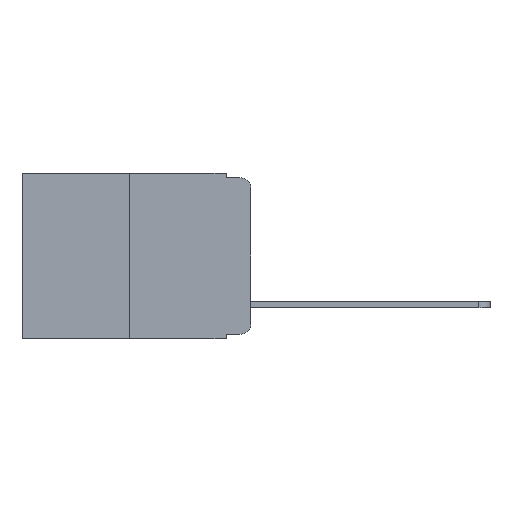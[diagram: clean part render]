
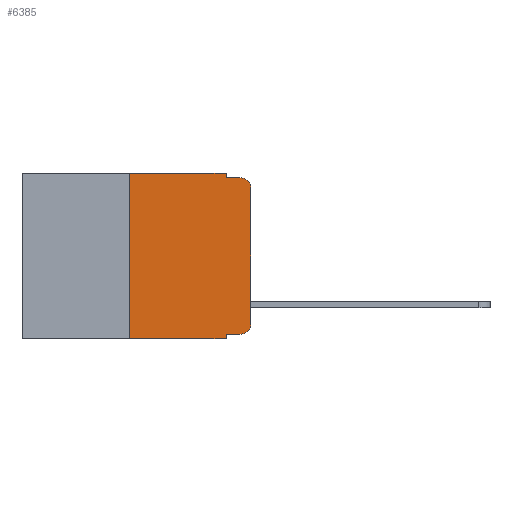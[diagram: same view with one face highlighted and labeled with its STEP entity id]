
A CAD part, left-side view. The second image highlights one B-rep face of the part: STEP entity #6385.
In plain terms, the highlighted planar face has unit normal (-1, 0, 0).
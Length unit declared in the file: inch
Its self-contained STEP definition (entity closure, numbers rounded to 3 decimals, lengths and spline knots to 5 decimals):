
#114 = VECTOR ( 'NONE', #10742, 39.37008 ) ;
#487 = ORIENTED_EDGE ( 'NONE', *, *, #7247, .T. ) ;
#564 = ORIENTED_EDGE ( 'NONE', *, *, #7189, .T. ) ;
#660 = ORIENTED_EDGE ( 'NONE', *, *, #6929, .F. ) ;
#783 = VERTEX_POINT ( 'NONE', #8067 ) ;
#1077 = ORIENTED_EDGE ( 'NONE', *, *, #7345, .T. ) ;
#1252 = ORIENTED_EDGE ( 'NONE', *, *, #6862, .F. ) ;
#1576 = VERTEX_POINT ( 'NONE', #7531 ) ;
#1654 = ORIENTED_EDGE ( 'NONE', *, *, #7230, .F. ) ;
#2025 = VERTEX_POINT ( 'NONE', #2436 ) ;
#2248 = DIRECTION ( 'NONE',  ( -1., 0., 0. ) ) ;
#2436 = CARTESIAN_POINT ( 'NONE',  ( 0., 0.02, -0.333 ) ) ;
#2529 = LINE ( 'NONE', #7719, #4609 ) ;
#2545 = ORIENTED_EDGE ( 'NONE', *, *, #6733, .F. ) ;
#2720 = CARTESIAN_POINT ( 'NONE',  ( 0., 0.051, 0. ) ) ;
#3143 = PLANE ( 'NONE',  #5312 ) ;
#3293 = CARTESIAN_POINT ( 'NONE',  ( 0., 0.051, -0.343 ) ) ;
#3547 = VECTOR ( 'NONE', #6724, 39.37008 ) ;
#3591 = ORIENTED_EDGE ( 'NONE', *, *, #5515, .T. ) ;
#3782 = AXIS2_PLACEMENT_3D ( 'NONE', #8034, #2248, #8924 ) ;
#3827 = DIRECTION ( 'NONE',  ( 0., 0., -1. ) ) ;
#4185 = VECTOR ( 'NONE', #3827, 39.37008 ) ;
#4446 = EDGE_LOOP ( 'NONE', ( #3591, #7866, #7164, #2545, #1654, #1252, #1077, #660, #564, #487 ) ) ;
#4468 = LINE ( 'NONE', #2720, #4185 ) ;
#4572 = VERTEX_POINT ( 'NONE', #9995 ) ;
#4609 = VECTOR ( 'NONE', #10327, 39.37008 ) ;
#4756 = LINE ( 'NONE', #7094, #9540 ) ;
#5075 = VECTOR ( 'NONE', #9643, 39.37008 ) ;
#5179 = DIRECTION ( 'NONE',  ( 0., 0., -1. ) ) ;
#5312 = AXIS2_PLACEMENT_3D ( 'NONE', #11291, #7882, #5179 ) ;
#5388 = LINE ( 'NONE', #6174, #5075 ) ;
#5488 = CARTESIAN_POINT ( 'NONE',  ( 0., 0.051, -0.01 ) ) ;
#5515 = EDGE_CURVE ( 'NONE', #6051, #1576, #6715, .T. ) ;
#5832 = LINE ( 'NONE', #9034, #114 ) ;
#5993 = DIRECTION ( 'NONE',  ( -1., 0., 0. ) ) ;
#6028 = VERTEX_POINT ( 'NONE', #11515 ) ;
#6043 = CARTESIAN_POINT ( 'NONE',  ( 0., 0.051, 0. ) ) ;
#6051 = VERTEX_POINT ( 'NONE', #8989 ) ;
#6174 = CARTESIAN_POINT ( 'NONE',  ( 0., 0.051, -0.333 ) ) ;
#6195 = EDGE_CURVE ( 'NONE', #1576, #6028, #8511, .T. ) ;
#6385 = ADVANCED_FACE ( 'NONE', ( #7403 ), #3143, .F. ) ;
#6624 = EDGE_CURVE ( 'NONE', #783, #6028, #12288, .T. ) ;
#6715 = LINE ( 'NONE', #11034, #10800 ) ;
#6724 = DIRECTION ( 'NONE',  ( 0., 0., 1. ) ) ;
#6733 = EDGE_CURVE ( 'NONE', #8177, #783, #4468, .T. ) ;
#6862 = EDGE_CURVE ( 'NONE', #7215, #4572, #10773, .T. ) ;
#6929 = EDGE_CURVE ( 'NONE', #12127, #11826, #2529, .T. ) ;
#7094 = CARTESIAN_POINT ( 'NONE',  ( 0., 0.473, 0. ) ) ;
#7164 = ORIENTED_EDGE ( 'NONE', *, *, #6624, .F. ) ;
#7189 = EDGE_CURVE ( 'NONE', #12127, #2025, #5388, .T. ) ;
#7215 = VERTEX_POINT ( 'NONE', #10550 ) ;
#7230 = EDGE_CURVE ( 'NONE', #4572, #8177, #4756, .T. ) ;
#7247 = EDGE_CURVE ( 'NONE', #2025, #6051, #9036, .T. ) ;
#7345 = EDGE_CURVE ( 'NONE', #7215, #11826, #5832, .T. ) ;
#7403 = FACE_OUTER_BOUND ( 'NONE', #4446, .T. ) ;
#7531 = CARTESIAN_POINT ( 'NONE',  ( 0., 0., -0.03 ) ) ;
#7612 = DIRECTION ( 'NONE',  ( 0., 0., 1. ) ) ;
#7719 = CARTESIAN_POINT ( 'NONE',  ( 0., 0.051, 0. ) ) ;
#7866 = ORIENTED_EDGE ( 'NONE', *, *, #6195, .T. ) ;
#7882 = DIRECTION ( 'NONE',  ( 1., 0., 0. ) ) ;
#7997 = DIRECTION ( 'NONE',  ( 0., -1., 0. ) ) ;
#8034 = CARTESIAN_POINT ( 'NONE',  ( 0., 0.02, -0.313 ) ) ;
#8067 = CARTESIAN_POINT ( 'NONE',  ( 0., 0.051, -0.01 ) ) ;
#8177 = VERTEX_POINT ( 'NONE', #6043 ) ;
#8511 = CIRCLE ( 'NONE', #10858, 0.02 ) ;
#8924 = DIRECTION ( 'NONE',  ( 0., 0., -1. ) ) ;
#8989 = CARTESIAN_POINT ( 'NONE',  ( 0., 0., -0.313 ) ) ;
#9034 = CARTESIAN_POINT ( 'NONE',  ( 0., 0.473, -0.343 ) ) ;
#9036 = CIRCLE ( 'NONE', #3782, 0.02 ) ;
#9540 = VECTOR ( 'NONE', #7997, 39.37008 ) ;
#9643 = DIRECTION ( 'NONE',  ( 0., -1., 0. ) ) ;
#9995 = CARTESIAN_POINT ( 'NONE',  ( 0., 0.25, 0. ) ) ;
#10213 = CARTESIAN_POINT ( 'NONE',  ( 0., 0.25, 0. ) ) ;
#10327 = DIRECTION ( 'NONE',  ( 0., 0., -1. ) ) ;
#10550 = CARTESIAN_POINT ( 'NONE',  ( 0., 0.25, -0.343 ) ) ;
#10742 = DIRECTION ( 'NONE',  ( 0., -1., 0. ) ) ;
#10773 = LINE ( 'NONE', #10213, #3547 ) ;
#10800 = VECTOR ( 'NONE', #7612, 39.37008 ) ;
#10858 = AXIS2_PLACEMENT_3D ( 'NONE', #11185, #5993, #11984 ) ;
#11034 = CARTESIAN_POINT ( 'NONE',  ( 0., 0., 0. ) ) ;
#11185 = CARTESIAN_POINT ( 'NONE',  ( 0., 0.02, -0.03 ) ) ;
#11291 = CARTESIAN_POINT ( 'NONE',  ( 0., 0.473, 0. ) ) ;
#11515 = CARTESIAN_POINT ( 'NONE',  ( 0., 0.02, -0.01 ) ) ;
#11564 = DIRECTION ( 'NONE',  ( 0., -1., 0. ) ) ;
#11672 = CARTESIAN_POINT ( 'NONE',  ( 0., 0.051, -0.333 ) ) ;
#11826 = VERTEX_POINT ( 'NONE', #3293 ) ;
#11984 = DIRECTION ( 'NONE',  ( 0., 0., -1. ) ) ;
#12033 = VECTOR ( 'NONE', #11564, 39.37008 ) ;
#12127 = VERTEX_POINT ( 'NONE', #11672 ) ;
#12288 = LINE ( 'NONE', #5488, #12033 ) ;
